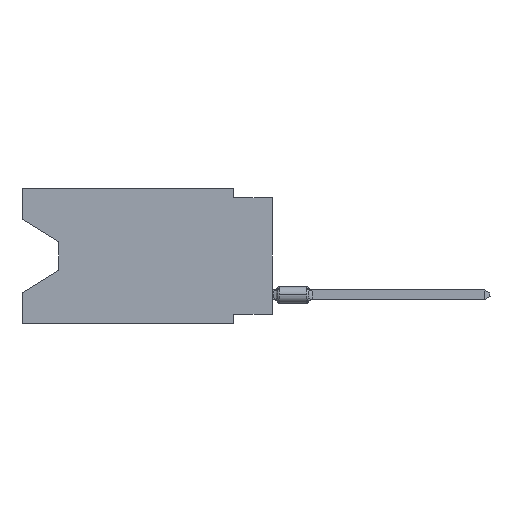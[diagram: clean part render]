
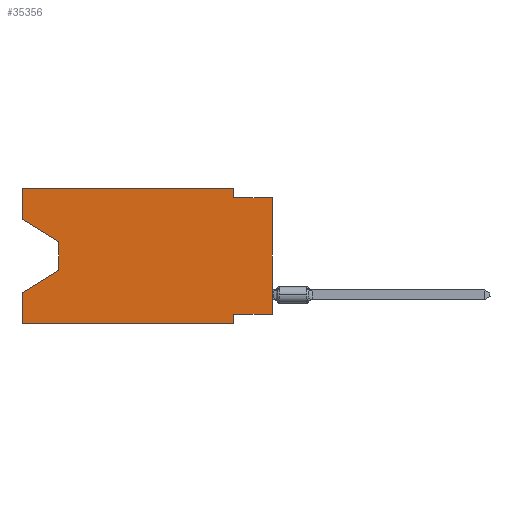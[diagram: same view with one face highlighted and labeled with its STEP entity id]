
A CAD part, left-side view. The second image highlights one B-rep face of the part: STEP entity #35356.
In plain terms, the highlighted planar face has unit normal (-1, 0, 0).
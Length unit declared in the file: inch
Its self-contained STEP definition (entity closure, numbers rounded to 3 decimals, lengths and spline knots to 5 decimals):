
#64 = CARTESIAN_POINT ( 'NONE',  ( 0., 0., 0. ) ) ;
#477 = CARTESIAN_POINT ( 'NONE',  ( 0., 0., -0.025 ) ) ;
#981 = EDGE_CURVE ( 'NONE', #21497, #29766, #23608, .T. ) ;
#1171 = DIRECTION ( 'NONE',  ( 0., -0.855, -0.519 ) ) ;
#1352 = VECTOR ( 'NONE', #38093, 39.37008 ) ;
#2378 = LINE ( 'NONE', #41479, #36796 ) ;
#2416 = DIRECTION ( 'NONE',  ( 0., -1., 0. ) ) ;
#2523 = VECTOR ( 'NONE', #32603, 39.37008 ) ;
#5125 = DIRECTION ( 'NONE',  ( 0., 0., 1. ) ) ;
#6135 = VECTOR ( 'NONE', #61933, 39.37008 ) ;
#6873 = ORIENTED_EDGE ( 'NONE', *, *, #28086, .F. ) ;
#7043 = VECTOR ( 'NONE', #57932, 39.37008 ) ;
#7129 = CARTESIAN_POINT ( 'NONE',  ( 0., 0.645, 0. ) ) ;
#7565 = VERTEX_POINT ( 'NONE', #48446 ) ;
#7678 = DIRECTION ( 'NONE',  ( 0., 0., -1. ) ) ;
#8553 = FACE_OUTER_BOUND ( 'NONE', #14919, .T. ) ;
#9442 = CARTESIAN_POINT ( 'NONE',  ( 0., 0.1, -0.35 ) ) ;
#10642 = EDGE_CURVE ( 'NONE', #59870, #58078, #50846, .T. ) ;
#11926 = VECTOR ( 'NONE', #67318, 39.37008 ) ;
#13395 = CARTESIAN_POINT ( 'NONE',  ( 0., 0.55, -0.212 ) ) ;
#13775 = ORIENTED_EDGE ( 'NONE', *, *, #17328, .F. ) ;
#14144 = CARTESIAN_POINT ( 'NONE',  ( 0., 0.55, -0.138 ) ) ;
#14196 = LINE ( 'NONE', #19942, #7043 ) ;
#14919 = EDGE_LOOP ( 'NONE', ( #50960, #57792, #38458, #13775, #67003, #25304, #6873, #47323, #45912, #53952, #29906, #16014 ) ) ;
#16014 = ORIENTED_EDGE ( 'NONE', *, *, #54900, .F. ) ;
#16564 = LINE ( 'NONE', #40454, #39054 ) ;
#17328 = EDGE_CURVE ( 'NONE', #18602, #29766, #43503, .T. ) ;
#18458 = CARTESIAN_POINT ( 'NONE',  ( 0., 0.1, -0.35 ) ) ;
#18602 = VERTEX_POINT ( 'NONE', #38139 ) ;
#19046 = CARTESIAN_POINT ( 'NONE',  ( 0., 0.645, -0.08025 ) ) ;
#19942 = CARTESIAN_POINT ( 'NONE',  ( 0., 0., -0.025 ) ) ;
#21497 = VERTEX_POINT ( 'NONE', #13395 ) ;
#23608 = LINE ( 'NONE', #45472, #11926 ) ;
#24793 = CARTESIAN_POINT ( 'NONE',  ( 0., 0., -0.325 ) ) ;
#25304 = ORIENTED_EDGE ( 'NONE', *, *, #37477, .F. ) ;
#25702 = LINE ( 'NONE', #63681, #63137 ) ;
#25939 = LINE ( 'NONE', #64, #1352 ) ;
#27704 = VERTEX_POINT ( 'NONE', #49030 ) ;
#28086 = EDGE_CURVE ( 'NONE', #41394, #7565, #65778, .T. ) ;
#29718 = VECTOR ( 'NONE', #7678, 39.37008 ) ;
#29766 = VERTEX_POINT ( 'NONE', #37745 ) ;
#29906 = ORIENTED_EDGE ( 'NONE', *, *, #10642, .F. ) ;
#29996 = DIRECTION ( 'NONE',  ( 0., 0., -1. ) ) ;
#31077 = DIRECTION ( 'NONE',  ( 0., 0., -1. ) ) ;
#31580 = VERTEX_POINT ( 'NONE', #19046 ) ;
#32603 = DIRECTION ( 'NONE',  ( 0., 0., 1. ) ) ;
#35356 = ADVANCED_FACE ( 'NONE', ( #8553 ), #67013, .F. ) ;
#36796 = VECTOR ( 'NONE', #31077, 39.37008 ) ;
#37346 = CARTESIAN_POINT ( 'NONE',  ( 0., 0.645, 0. ) ) ;
#37477 = EDGE_CURVE ( 'NONE', #7565, #41024, #56466, .T. ) ;
#37745 = CARTESIAN_POINT ( 'NONE',  ( 0., 0.645, -0.26975 ) ) ;
#38093 = DIRECTION ( 'NONE',  ( 0., 0., 1. ) ) ;
#38139 = CARTESIAN_POINT ( 'NONE',  ( 0., 0.645, -0.35 ) ) ;
#38458 = ORIENTED_EDGE ( 'NONE', *, *, #981, .T. ) ;
#38857 = EDGE_CURVE ( 'NONE', #18602, #41024, #16564, .T. ) ;
#39054 = VECTOR ( 'NONE', #2416, 39.37008 ) ;
#39404 = EDGE_CURVE ( 'NONE', #27704, #50595, #14196, .T. ) ;
#39878 = EDGE_CURVE ( 'NONE', #41394, #50595, #25939, .T. ) ;
#40454 = CARTESIAN_POINT ( 'NONE',  ( 0., 0.645, -0.35 ) ) ;
#41024 = VERTEX_POINT ( 'NONE', #9442 ) ;
#41394 = VERTEX_POINT ( 'NONE', #24793 ) ;
#41479 = CARTESIAN_POINT ( 'NONE',  ( 0., 0.55, -0.138 ) ) ;
#43503 = LINE ( 'NONE', #69321, #54764 ) ;
#43938 = CARTESIAN_POINT ( 'NONE',  ( 0., 0.1, 0. ) ) ;
#45472 = CARTESIAN_POINT ( 'NONE',  ( 0., 0.55, -0.212 ) ) ;
#45588 = VECTOR ( 'NONE', #59001, 39.37008 ) ;
#45912 = ORIENTED_EDGE ( 'NONE', *, *, #39404, .F. ) ;
#47323 = ORIENTED_EDGE ( 'NONE', *, *, #39878, .T. ) ;
#48446 = CARTESIAN_POINT ( 'NONE',  ( 0., 0.1, -0.325 ) ) ;
#49030 = CARTESIAN_POINT ( 'NONE',  ( 0., 0.1, -0.025 ) ) ;
#50595 = VERTEX_POINT ( 'NONE', #477 ) ;
#50719 = EDGE_CURVE ( 'NONE', #31580, #62653, #61415, .T. ) ;
#50846 = LINE ( 'NONE', #62643, #6135 ) ;
#50891 = DIRECTION ( 'NONE',  ( 1., 0., 0. ) ) ;
#50960 = ORIENTED_EDGE ( 'NONE', *, *, #50719, .T. ) ;
#53952 = ORIENTED_EDGE ( 'NONE', *, *, #65652, .F. ) ;
#54764 = VECTOR ( 'NONE', #5125, 39.37008 ) ;
#54900 = EDGE_CURVE ( 'NONE', #31580, #59870, #65920, .T. ) ;
#56052 = CARTESIAN_POINT ( 'NONE',  ( 0., 0.645, -0.08025 ) ) ;
#56466 = LINE ( 'NONE', #18458, #29718 ) ;
#57792 = ORIENTED_EDGE ( 'NONE', *, *, #66779, .T. ) ;
#57932 = DIRECTION ( 'NONE',  ( 0., -1., 0. ) ) ;
#58078 = VERTEX_POINT ( 'NONE', #43938 ) ;
#59001 = DIRECTION ( 'NONE',  ( 0., 1., 0. ) ) ;
#59485 = CARTESIAN_POINT ( 'NONE',  ( 0., 0.645, 0. ) ) ;
#59870 = VERTEX_POINT ( 'NONE', #37346 ) ;
#61415 = LINE ( 'NONE', #56052, #69808 ) ;
#61933 = DIRECTION ( 'NONE',  ( 0., -1., 0. ) ) ;
#62643 = CARTESIAN_POINT ( 'NONE',  ( 0., 0.645, 0. ) ) ;
#62653 = VERTEX_POINT ( 'NONE', #14144 ) ;
#63137 = VECTOR ( 'NONE', #29996, 39.37008 ) ;
#63681 = CARTESIAN_POINT ( 'NONE',  ( 0., 0.1, 0. ) ) ;
#64992 = AXIS2_PLACEMENT_3D ( 'NONE', #7129, #50891, #67352 ) ;
#65652 = EDGE_CURVE ( 'NONE', #58078, #27704, #25702, .T. ) ;
#65778 = LINE ( 'NONE', #70787, #45588 ) ;
#65920 = LINE ( 'NONE', #59485, #2523 ) ;
#66779 = EDGE_CURVE ( 'NONE', #62653, #21497, #2378, .T. ) ;
#67003 = ORIENTED_EDGE ( 'NONE', *, *, #38857, .T. ) ;
#67013 = PLANE ( 'NONE',  #64992 ) ;
#67318 = DIRECTION ( 'NONE',  ( 0., 0.855, -0.519 ) ) ;
#67352 = DIRECTION ( 'NONE',  ( 0., 0., -1. ) ) ;
#69321 = CARTESIAN_POINT ( 'NONE',  ( 0., 0.645, 0. ) ) ;
#69808 = VECTOR ( 'NONE', #1171, 39.37008 ) ;
#70787 = CARTESIAN_POINT ( 'NONE',  ( 0., 0., -0.325 ) ) ;
